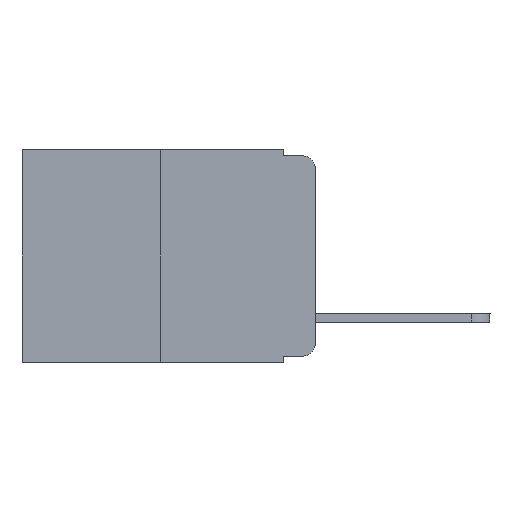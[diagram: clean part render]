
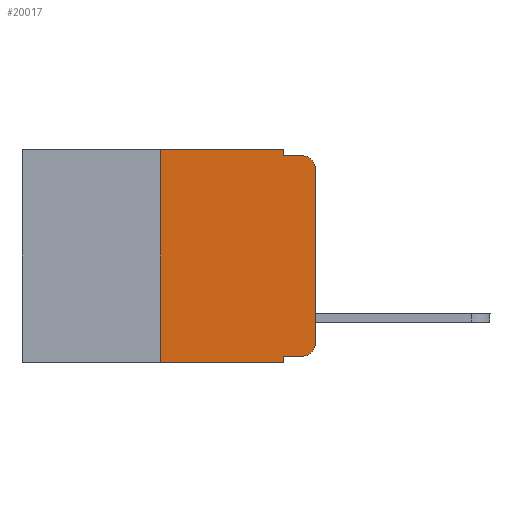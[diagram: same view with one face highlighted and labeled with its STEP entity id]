
A CAD part, left-side view. The second image highlights one B-rep face of the part: STEP entity #20017.
In plain terms, the highlighted planar face has unit normal (-1, 0, 0).
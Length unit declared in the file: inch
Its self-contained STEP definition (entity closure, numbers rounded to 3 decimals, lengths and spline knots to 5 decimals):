
#917 = CARTESIAN_POINT ( 'NONE',  ( 0., 0.051, -0.01 ) ) ;
#1006 = DIRECTION ( 'NONE',  ( 0., 0., -1. ) ) ;
#1107 = CARTESIAN_POINT ( 'NONE',  ( 0., 0.051, 0. ) ) ;
#1763 = VECTOR ( 'NONE', #20175, 39.37008 ) ;
#1859 = LINE ( 'NONE', #12977, #19844 ) ;
#2600 = ORIENTED_EDGE ( 'NONE', *, *, #14852, .F. ) ;
#2747 = LINE ( 'NONE', #8654, #16486 ) ;
#3580 = CARTESIAN_POINT ( 'NONE',  ( 0., 0.051, 0. ) ) ;
#3717 = CARTESIAN_POINT ( 'NONE',  ( 0., 0.02, -0.03 ) ) ;
#3747 = ORIENTED_EDGE ( 'NONE', *, *, #17977, .T. ) ;
#3903 = ORIENTED_EDGE ( 'NONE', *, *, #7999, .F. ) ;
#3955 = EDGE_CURVE ( 'NONE', #17197, #10837, #20565, .T. ) ;
#4044 = EDGE_CURVE ( 'NONE', #17764, #9427, #7234, .T. ) ;
#4182 = CARTESIAN_POINT ( 'NONE',  ( 0., 0., 0. ) ) ;
#5004 = ORIENTED_EDGE ( 'NONE', *, *, #6670, .T. ) ;
#5352 = EDGE_CURVE ( 'NONE', #19643, #17197, #7699, .T. ) ;
#5410 = VERTEX_POINT ( 'NONE', #18965 ) ;
#5873 = LINE ( 'NONE', #10222, #19448 ) ;
#5953 = AXIS2_PLACEMENT_3D ( 'NONE', #15677, #12823, #6304 ) ;
#6046 = CARTESIAN_POINT ( 'NONE',  ( 0., 0.02, -0.313 ) ) ;
#6304 = DIRECTION ( 'NONE',  ( 0., 0., -1. ) ) ;
#6497 = PLANE ( 'NONE',  #5953 ) ;
#6670 = EDGE_CURVE ( 'NONE', #19388, #19643, #10224, .T. ) ;
#7146 = CARTESIAN_POINT ( 'NONE',  ( 0., 0.473, -0.343 ) ) ;
#7234 = LINE ( 'NONE', #1107, #7262 ) ;
#7262 = VECTOR ( 'NONE', #1006, 39.37008 ) ;
#7394 = DIRECTION ( 'NONE',  ( 0., 0., -1. ) ) ;
#7444 = VECTOR ( 'NONE', #19602, 39.37008 ) ;
#7699 = LINE ( 'NONE', #4182, #18959 ) ;
#7718 = CARTESIAN_POINT ( 'NONE',  ( 0., 0., -0.03 ) ) ;
#7999 = EDGE_CURVE ( 'NONE', #8405, #5410, #5873, .T. ) ;
#8280 = DIRECTION ( 'NONE',  ( 0., 0., -1. ) ) ;
#8405 = VERTEX_POINT ( 'NONE', #18147 ) ;
#8475 = DIRECTION ( 'NONE',  ( -1., 0., 0. ) ) ;
#8654 = CARTESIAN_POINT ( 'NONE',  ( 0., 0.473, 0. ) ) ;
#9076 = ORIENTED_EDGE ( 'NONE', *, *, #15488, .F. ) ;
#9427 = VERTEX_POINT ( 'NONE', #11449 ) ;
#9951 = LINE ( 'NONE', #7146, #12842 ) ;
#10222 = CARTESIAN_POINT ( 'NONE',  ( 0., 0.25, 0. ) ) ;
#10224 = CIRCLE ( 'NONE', #12888, 0.02 ) ;
#10837 = VERTEX_POINT ( 'NONE', #11504 ) ;
#10895 = CARTESIAN_POINT ( 'NONE',  ( 0., 0.02, -0.333 ) ) ;
#10925 = VERTEX_POINT ( 'NONE', #14740 ) ;
#11449 = CARTESIAN_POINT ( 'NONE',  ( 0., 0.051, -0.01 ) ) ;
#11504 = CARTESIAN_POINT ( 'NONE',  ( 0., 0.02, -0.01 ) ) ;
#11544 = ORIENTED_EDGE ( 'NONE', *, *, #12247, .T. ) ;
#12247 = EDGE_CURVE ( 'NONE', #8405, #15652, #9951, .T. ) ;
#12365 = CARTESIAN_POINT ( 'NONE',  ( 0., 0.051, 0. ) ) ;
#12443 = ORIENTED_EDGE ( 'NONE', *, *, #4044, .F. ) ;
#12552 = CARTESIAN_POINT ( 'NONE',  ( 0., 0., -0.313 ) ) ;
#12716 = LINE ( 'NONE', #3580, #7444 ) ;
#12823 = DIRECTION ( 'NONE',  ( 1., 0., 0. ) ) ;
#12842 = VECTOR ( 'NONE', #19550, 39.37008 ) ;
#12888 = AXIS2_PLACEMENT_3D ( 'NONE', #6046, #18666, #7394 ) ;
#12977 = CARTESIAN_POINT ( 'NONE',  ( 0., 0.051, -0.333 ) ) ;
#13451 = DIRECTION ( 'NONE',  ( 0., 0., 1. ) ) ;
#13942 = DIRECTION ( 'NONE',  ( 0., 0., 1. ) ) ;
#14740 = CARTESIAN_POINT ( 'NONE',  ( 0., 0.051, -0.333 ) ) ;
#14852 = EDGE_CURVE ( 'NONE', #9427, #10837, #15491, .T. ) ;
#15488 = EDGE_CURVE ( 'NONE', #10925, #15652, #12716, .T. ) ;
#15491 = LINE ( 'NONE', #917, #1763 ) ;
#15602 = AXIS2_PLACEMENT_3D ( 'NONE', #3717, #8475, #8280 ) ;
#15652 = VERTEX_POINT ( 'NONE', #18155 ) ;
#15677 = CARTESIAN_POINT ( 'NONE',  ( 0., 0.473, 0. ) ) ;
#15741 = ORIENTED_EDGE ( 'NONE', *, *, #5352, .T. ) ;
#16088 = FACE_OUTER_BOUND ( 'NONE', #20204, .T. ) ;
#16429 = ORIENTED_EDGE ( 'NONE', *, *, #3955, .T. ) ;
#16486 = VECTOR ( 'NONE', #19700, 39.37008 ) ;
#17060 = EDGE_CURVE ( 'NONE', #5410, #17764, #2747, .T. ) ;
#17197 = VERTEX_POINT ( 'NONE', #7718 ) ;
#17764 = VERTEX_POINT ( 'NONE', #12365 ) ;
#17977 = EDGE_CURVE ( 'NONE', #10925, #19388, #1859, .T. ) ;
#18147 = CARTESIAN_POINT ( 'NONE',  ( 0., 0.25, -0.343 ) ) ;
#18155 = CARTESIAN_POINT ( 'NONE',  ( 0., 0.051, -0.343 ) ) ;
#18666 = DIRECTION ( 'NONE',  ( -1., 0., 0. ) ) ;
#18959 = VECTOR ( 'NONE', #13942, 39.37008 ) ;
#18965 = CARTESIAN_POINT ( 'NONE',  ( 0., 0.25, 0. ) ) ;
#19056 = ORIENTED_EDGE ( 'NONE', *, *, #17060, .F. ) ;
#19358 = DIRECTION ( 'NONE',  ( 0., -1., 0. ) ) ;
#19388 = VERTEX_POINT ( 'NONE', #10895 ) ;
#19448 = VECTOR ( 'NONE', #13451, 39.37008 ) ;
#19550 = DIRECTION ( 'NONE',  ( 0., -1., 0. ) ) ;
#19602 = DIRECTION ( 'NONE',  ( 0., 0., -1. ) ) ;
#19643 = VERTEX_POINT ( 'NONE', #12552 ) ;
#19700 = DIRECTION ( 'NONE',  ( 0., -1., 0. ) ) ;
#19844 = VECTOR ( 'NONE', #19358, 39.37008 ) ;
#20017 = ADVANCED_FACE ( 'NONE', ( #16088 ), #6497, .F. ) ;
#20175 = DIRECTION ( 'NONE',  ( 0., -1., 0. ) ) ;
#20204 = EDGE_LOOP ( 'NONE', ( #15741, #16429, #2600, #12443, #19056, #3903, #11544, #9076, #3747, #5004 ) ) ;
#20565 = CIRCLE ( 'NONE', #15602, 0.02 ) ;
